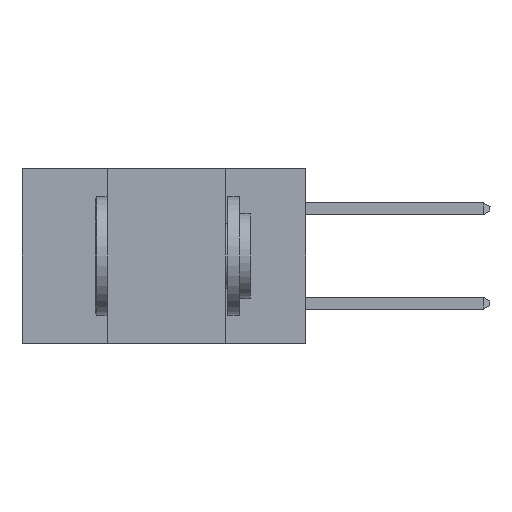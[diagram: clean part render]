
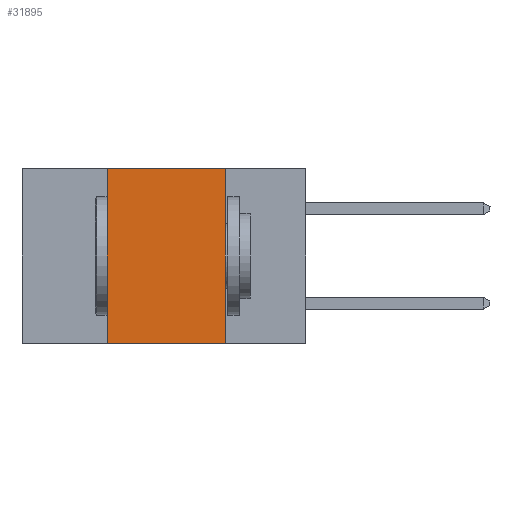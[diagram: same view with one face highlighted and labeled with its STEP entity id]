
A CAD part, left-side view. The second image highlights one B-rep face of the part: STEP entity #31895.
In plain terms, the highlighted planar face has unit normal (-1, 0, 0).
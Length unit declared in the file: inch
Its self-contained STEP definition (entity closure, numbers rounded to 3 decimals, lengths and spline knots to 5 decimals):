
#236 = DIRECTION ( 'NONE',  ( 1., 0., 0. ) ) ;
#353 = EDGE_CURVE ( 'NONE', #19318, #24294, #16808, .T. ) ;
#357 = ORIENTED_EDGE ( 'NONE', *, *, #353, .F. ) ;
#2412 = DIRECTION ( 'NONE',  ( 0., 0., -1. ) ) ;
#4859 = DIRECTION ( 'NONE',  ( 0., 0., 1. ) ) ;
#5099 = PLANE ( 'NONE',  #29593 ) ;
#6048 = VECTOR ( 'NONE', #22333, 39.37008 ) ;
#6195 = LINE ( 'NONE', #18277, #9607 ) ;
#6452 = VERTEX_POINT ( 'NONE', #14299 ) ;
#7037 = CARTESIAN_POINT ( 'NONE',  ( 0., 0.42, -0.37 ) ) ;
#8882 = LINE ( 'NONE', #24728, #25199 ) ;
#9036 = CARTESIAN_POINT ( 'NONE',  ( 0., 0.42, 0. ) ) ;
#9607 = VECTOR ( 'NONE', #20675, 39.37008 ) ;
#14044 = CARTESIAN_POINT ( 'NONE',  ( 0., 0.42, 0. ) ) ;
#14299 = CARTESIAN_POINT ( 'NONE',  ( 0., 0.17, -0.37 ) ) ;
#16808 = LINE ( 'NONE', #24531, #6048 ) ;
#16986 = LINE ( 'NONE', #14044, #29045 ) ;
#18277 = CARTESIAN_POINT ( 'NONE',  ( 0., 0.6, -0.37 ) ) ;
#19318 = VERTEX_POINT ( 'NONE', #9036 ) ;
#20675 = DIRECTION ( 'NONE',  ( 0., -1., 0. ) ) ;
#21447 = EDGE_LOOP ( 'NONE', ( #21617, #357, #22226, #29788 ) ) ;
#21617 = ORIENTED_EDGE ( 'NONE', *, *, #24596, .F. ) ;
#22226 = ORIENTED_EDGE ( 'NONE', *, *, #30516, .F. ) ;
#22333 = DIRECTION ( 'NONE',  ( 0., -1., 0. ) ) ;
#22877 = VERTEX_POINT ( 'NONE', #7037 ) ;
#24294 = VERTEX_POINT ( 'NONE', #30553 ) ;
#24531 = CARTESIAN_POINT ( 'NONE',  ( 0., 0.6, 0. ) ) ;
#24596 = EDGE_CURVE ( 'NONE', #24294, #6452, #8882, .T. ) ;
#24728 = CARTESIAN_POINT ( 'NONE',  ( 0., 0.17, 0. ) ) ;
#24910 = EDGE_CURVE ( 'NONE', #22877, #6452, #6195, .T. ) ;
#24948 = CARTESIAN_POINT ( 'NONE',  ( 0., 0.6, 0. ) ) ;
#25199 = VECTOR ( 'NONE', #2412, 39.37008 ) ;
#29045 = VECTOR ( 'NONE', #4859, 39.37008 ) ;
#29593 = AXIS2_PLACEMENT_3D ( 'NONE', #24948, #236, #32091 ) ;
#29788 = ORIENTED_EDGE ( 'NONE', *, *, #24910, .T. ) ;
#29839 = FACE_OUTER_BOUND ( 'NONE', #21447, .T. ) ;
#30516 = EDGE_CURVE ( 'NONE', #22877, #19318, #16986, .T. ) ;
#30553 = CARTESIAN_POINT ( 'NONE',  ( 0., 0.17, 0. ) ) ;
#31895 = ADVANCED_FACE ( 'NONE', ( #29839 ), #5099, .F. ) ;
#32091 = DIRECTION ( 'NONE',  ( 0., 0., -1. ) ) ;
